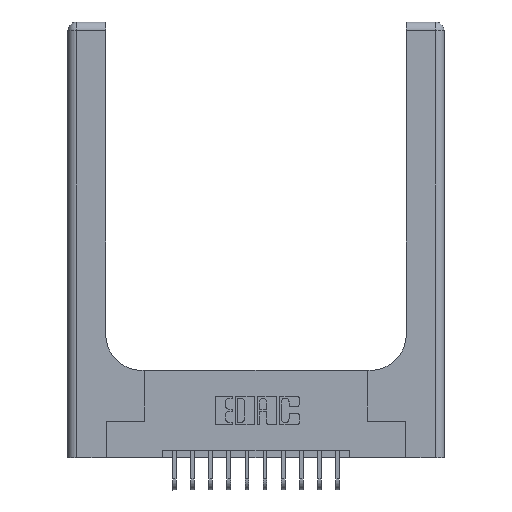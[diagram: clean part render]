
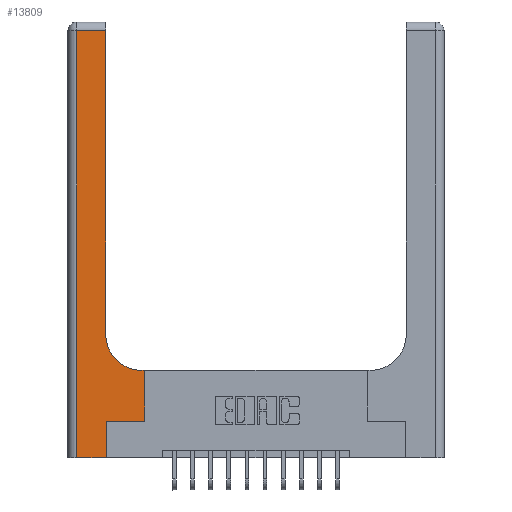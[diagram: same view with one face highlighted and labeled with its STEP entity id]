
A CAD part, top view. The second image highlights one B-rep face of the part: STEP entity #13809.
In plain terms, the highlighted planar face has unit normal (0, 0, 1).
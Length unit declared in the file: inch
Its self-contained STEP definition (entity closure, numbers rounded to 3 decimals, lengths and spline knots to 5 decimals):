
#163 = VERTEX_POINT ( 'NONE', #10530 ) ;
#200 = EDGE_CURVE ( 'NONE', #3643, #1803, #6014, .T. ) ;
#510 = DIRECTION ( 'NONE',  ( 0., -1., 0. ) ) ;
#913 = ORIENTED_EDGE ( 'NONE', *, *, #16906, .T. ) ;
#1204 = VECTOR ( 'NONE', #15873, 39.37008 ) ;
#1210 = CARTESIAN_POINT ( 'NONE',  ( 0.06, 0., 0.37 ) ) ;
#1689 = VERTEX_POINT ( 'NONE', #6714 ) ;
#1803 = VERTEX_POINT ( 'NONE', #17162 ) ;
#2240 = CARTESIAN_POINT ( 'NONE',  ( 0.26, 0.85, 0.37 ) ) ;
#2299 = CARTESIAN_POINT ( 'NONE',  ( 0., 0., 0.37 ) ) ;
#2846 = CARTESIAN_POINT ( 'NONE',  ( 0.26, 0.6, 0.37 ) ) ;
#2997 = ORIENTED_EDGE ( 'NONE', *, *, #11809, .T. ) ;
#3378 = LINE ( 'NONE', #10723, #8517 ) ;
#3481 = LINE ( 'NONE', #4467, #15713 ) ;
#3643 = VERTEX_POINT ( 'NONE', #10893 ) ;
#4070 = VECTOR ( 'NONE', #16269, 39.37008 ) ;
#4230 = PLANE ( 'NONE',  #7898 ) ;
#4467 = CARTESIAN_POINT ( 'NONE',  ( 0.06, 3., 0.37 ) ) ;
#4521 = VERTEX_POINT ( 'NONE', #17357 ) ;
#4739 = EDGE_CURVE ( 'NONE', #15890, #163, #3378, .T. ) ;
#4886 = EDGE_CURVE ( 'NONE', #10492, #4521, #5503, .T. ) ;
#5208 = CARTESIAN_POINT ( 'NONE',  ( 0.528, 0.25, 0.37 ) ) ;
#5481 = DIRECTION ( 'NONE',  ( 1., 0., 0. ) ) ;
#5503 = LINE ( 'NONE', #2299, #1204 ) ;
#5602 = LINE ( 'NONE', #7074, #14143 ) ;
#5623 = CARTESIAN_POINT ( 'NONE',  ( 0., 3., 0.37 ) ) ;
#5905 = ORIENTED_EDGE ( 'NONE', *, *, #12095, .T. ) ;
#5909 = LINE ( 'NONE', #2846, #16206 ) ;
#6014 = LINE ( 'NONE', #11339, #4070 ) ;
#6101 = VERTEX_POINT ( 'NONE', #7329 ) ;
#6523 = DIRECTION ( 'NONE',  ( 0., 1., 0. ) ) ;
#6714 = CARTESIAN_POINT ( 'NONE',  ( 0.51, 0.6, 0.37 ) ) ;
#7074 = CARTESIAN_POINT ( 'NONE',  ( 0.265, 0.25, 0.37 ) ) ;
#7329 = CARTESIAN_POINT ( 'NONE',  ( 0.265, 0.25, 0.37 ) ) ;
#7898 = AXIS2_PLACEMENT_3D ( 'NONE', #5623, #15183, #16851 ) ;
#8312 = EDGE_CURVE ( 'NONE', #6101, #15890, #5602, .T. ) ;
#8517 = VECTOR ( 'NONE', #17776, 39.37008 ) ;
#8588 = CIRCLE ( 'NONE', #14059, 0.25 ) ;
#8801 = EDGE_LOOP ( 'NONE', ( #913, #14375, #2997, #12384, #5905, #17780, #15514, #14119, #10861 ) ) ;
#9840 = DIRECTION ( 'NONE',  ( 0., 1., 0. ) ) ;
#10277 = FACE_OUTER_BOUND ( 'NONE', #8801, .T. ) ;
#10492 = VERTEX_POINT ( 'NONE', #1210 ) ;
#10530 = CARTESIAN_POINT ( 'NONE',  ( 0.528, 0.6, 0.37 ) ) ;
#10538 = CARTESIAN_POINT ( 'NONE',  ( 0.265, 0., 0.37 ) ) ;
#10578 = EDGE_CURVE ( 'NONE', #163, #1689, #5909, .T. ) ;
#10715 = VECTOR ( 'NONE', #6523, 39.37008 ) ;
#10723 = CARTESIAN_POINT ( 'NONE',  ( 0.528, 0.25, 0.37 ) ) ;
#10779 = DIRECTION ( 'NONE',  ( 1., 0., 0. ) ) ;
#10861 = ORIENTED_EDGE ( 'NONE', *, *, #13858, .T. ) ;
#10893 = CARTESIAN_POINT ( 'NONE',  ( 0.26, 2.94, 0.37 ) ) ;
#11339 = CARTESIAN_POINT ( 'NONE',  ( 0., 2.94, 0.37 ) ) ;
#11809 = EDGE_CURVE ( 'NONE', #1803, #10492, #3481, .T. ) ;
#12095 = EDGE_CURVE ( 'NONE', #4521, #6101, #14822, .T. ) ;
#12384 = ORIENTED_EDGE ( 'NONE', *, *, #4886, .T. ) ;
#12446 = DIRECTION ( 'NONE',  ( -1., 0., 0. ) ) ;
#12944 = LINE ( 'NONE', #13918, #17339 ) ;
#13345 = VERTEX_POINT ( 'NONE', #2240 ) ;
#13415 = CARTESIAN_POINT ( 'NONE',  ( 0.51, 0.85, 0.37 ) ) ;
#13476 = DIRECTION ( 'NONE',  ( 0., 0., -1. ) ) ;
#13809 = ADVANCED_FACE ( 'NONE', ( #10277 ), #4230, .F. ) ;
#13858 = EDGE_CURVE ( 'NONE', #1689, #13345, #8588, .T. ) ;
#13918 = CARTESIAN_POINT ( 'NONE',  ( 0.26, 3., 0.37 ) ) ;
#14059 = AXIS2_PLACEMENT_3D ( 'NONE', #13415, #13476, #10779 ) ;
#14119 = ORIENTED_EDGE ( 'NONE', *, *, #10578, .T. ) ;
#14143 = VECTOR ( 'NONE', #5481, 39.37008 ) ;
#14375 = ORIENTED_EDGE ( 'NONE', *, *, #200, .T. ) ;
#14822 = LINE ( 'NONE', #10538, #10715 ) ;
#15183 = DIRECTION ( 'NONE',  ( 0., 0., -1. ) ) ;
#15514 = ORIENTED_EDGE ( 'NONE', *, *, #4739, .T. ) ;
#15713 = VECTOR ( 'NONE', #510, 39.37008 ) ;
#15873 = DIRECTION ( 'NONE',  ( 1., 0., 0. ) ) ;
#15890 = VERTEX_POINT ( 'NONE', #5208 ) ;
#16206 = VECTOR ( 'NONE', #12446, 39.37008 ) ;
#16269 = DIRECTION ( 'NONE',  ( -1., 0., 0. ) ) ;
#16851 = DIRECTION ( 'NONE',  ( -1., 0., 0. ) ) ;
#16906 = EDGE_CURVE ( 'NONE', #13345, #3643, #12944, .T. ) ;
#17162 = CARTESIAN_POINT ( 'NONE',  ( 0.06, 2.94, 0.37 ) ) ;
#17339 = VECTOR ( 'NONE', #9840, 39.37008 ) ;
#17357 = CARTESIAN_POINT ( 'NONE',  ( 0.265, 0., 0.37 ) ) ;
#17776 = DIRECTION ( 'NONE',  ( 0., 1., 0. ) ) ;
#17780 = ORIENTED_EDGE ( 'NONE', *, *, #8312, .T. ) ;
